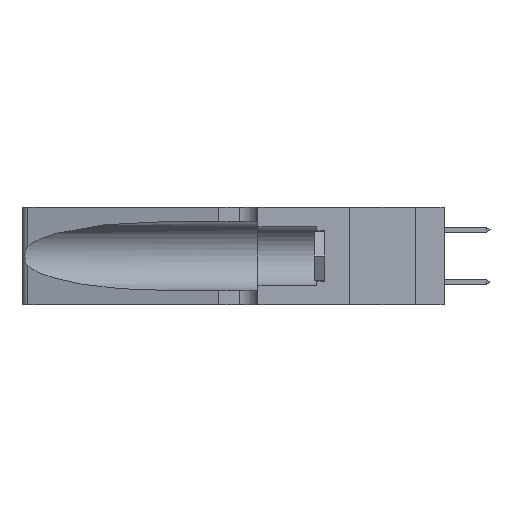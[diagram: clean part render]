
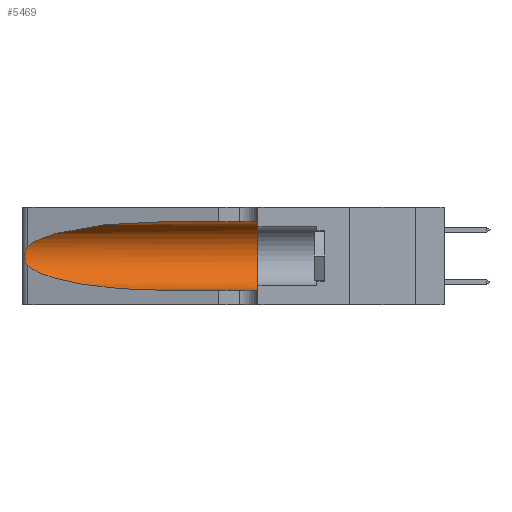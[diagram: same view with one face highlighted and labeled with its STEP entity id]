
A CAD part, left-side view. The second image highlights one B-rep face of the part: STEP entity #5469.
In plain terms, the highlighted cylindrical face has radius 3.308 mm (diameter 6.617 mm), a partial arc.
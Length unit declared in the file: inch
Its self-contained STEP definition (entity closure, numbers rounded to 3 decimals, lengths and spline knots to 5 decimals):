
#1336 = CARTESIAN_POINT ( 'NONE',  ( 0.1305, 1.61858, 0.185 ) ) ;
#1369 = ORIENTED_EDGE ( 'NONE', *, *, #7518, .T. ) ;
#2101 = DIRECTION ( 'NONE',  ( 0., -1., 0. ) ) ;
#2348 = EDGE_CURVE ( 'NONE', #13740, #12938, #23797, .T. ) ;
#2750 = CARTESIAN_POINT ( 'NONE',  ( 0.26018, 1.23835, 0.19895 ) ) ;
#2920 = CARTESIAN_POINT ( 'NONE',  ( 0.26017, 1.23833, 0.17102 ) ) ;
#3438 = CARTESIAN_POINT ( 'NONE',  ( 0.25487, 1.22718, 0.14631 ) ) ;
#4568 = EDGE_LOOP ( 'NONE', ( #7108, #1369, #13093, #8150, #4932, #17417 ) ) ;
#4824 = CARTESIAN_POINT ( 'NONE',  ( 0.25789, 1.23486, 0.15765 ) ) ;
#4932 = ORIENTED_EDGE ( 'NONE', *, *, #16822, .F. ) ;
#5037 = CARTESIAN_POINT ( 'NONE',  ( 0.25487, 1.22718, 0.22369 ) ) ;
#5038 = CARTESIAN_POINT ( 'NONE',  ( 0.1305, 0.72297, 0.05475 ) ) ;
#5103 = FACE_OUTER_BOUND ( 'NONE', #4568, .T. ) ;
#5469 = ADVANCED_FACE ( 'NONE', ( #5103 ), #8925, .F. ) ;
#5635 = DIRECTION ( 'NONE',  ( 0., -1., 0. ) ) ;
#6084 = VERTEX_POINT ( 'NONE', #10677 ) ;
#6521 = CARTESIAN_POINT ( 'NONE',  ( 0.25555, 1.22993, 0.14849 ) ) ;
#6771 = CARTESIAN_POINT ( 'NONE',  ( 0.25555, 1.22994, 0.2215 ) ) ;
#6838 = CARTESIAN_POINT ( 'NONE',  ( 0.1305, 0.35, 0.185 ) ) ;
#7108 = ORIENTED_EDGE ( 'NONE', *, *, #14461, .T. ) ;
#7281 = CARTESIAN_POINT ( 'NONE',  ( 0.25487, 1.22718, 0.22369 ) ) ;
#7518 = EDGE_CURVE ( 'NONE', #20914, #13740, #15071, .T. ) ;
#8150 = ORIENTED_EDGE ( 'NONE', *, *, #19286, .T. ) ;
#8511 = CARTESIAN_POINT ( 'NONE',  ( 0.18966, 0.96281, 0.31525 ) ) ;
#8925 = CYLINDRICAL_SURFACE ( 'NONE', #18607, 0.13025 ) ;
#10263 = CARTESIAN_POINT ( 'NONE',  ( 0.25487, 1.22718, 0.14631 ) ) ;
#10335 = AXIS2_PLACEMENT_3D ( 'NONE', #6838, #19932, #12716 ) ;
#10415 = CARTESIAN_POINT ( 'NONE',  ( 0.25854, 1.2359, 0.20912 ) ) ;
#10574 = CARTESIAN_POINT ( 'NONE',  ( 0.25639, 1.23184, 0.21858 ) ) ;
#10677 = CARTESIAN_POINT ( 'NONE',  ( 0.1305, 0.35, 0.05475 ) ) ;
#10706 = DIRECTION ( 'NONE',  ( 0., 0., -1. ) ) ;
#12007 = VERTEX_POINT ( 'NONE', #15693 ) ;
#12307 = CARTESIAN_POINT ( 'NONE',  ( 0.26075, 1.23896, 0.19203 ) ) ;
#12484 = CARTESIAN_POINT ( 'NONE',  ( 0.26075, 1.23896, 0.178 ) ) ;
#12716 = DIRECTION ( 'NONE',  ( 0., 0., 1. ) ) ;
#12938 = VERTEX_POINT ( 'NONE', #5038 ) ;
#13093 = ORIENTED_EDGE ( 'NONE', *, *, #2348, .T. ) ;
#13740 = VERTEX_POINT ( 'NONE', #3438 ) ;
#13821 = CIRCLE ( 'NONE', #10335, 0.13025 ) ;
#14421 = CARTESIAN_POINT ( 'NONE',  ( 0.18966, 0.96281, 0.05475 ) ) ;
#14461 = EDGE_CURVE ( 'NONE', #12007, #20914, #16277, .T. ) ;
#14545 = VECTOR ( 'NONE', #5635, 39.37008 ) ;
#15071 = B_SPLINE_CURVE_WITH_KNOTS ( 'NONE', 3,
 ( #21579, #6771, #10574, #23719, #10415, #2750, #12307, #12484, #2920, #23475, #4824, #23640, #6521, #10263 ),
 .UNSPECIFIED., .F., .F.,
 ( 4, 2, 2, 2, 2, 2, 4 ),
 ( 0., 0.00027, 0.00053, 0.00107, 0.0016, 0.00187, 0.00214 ),
 .UNSPECIFIED. ) ;
#15334 = VERTEX_POINT ( 'NONE', #21741 ) ;
#15693 = CARTESIAN_POINT ( 'NONE',  ( 0.1305, 0.72297, 0.31525 ) ) ;
#16277 =( BOUNDED_CURVE ( )  B_SPLINE_CURVE ( 3, ( #19763, #8511, #23928, #5037 ),
 .UNSPECIFIED., .F., .T. ) 
 B_SPLINE_CURVE_WITH_KNOTS ( ( 4, 4 ),
 ( 1.5708, 2.84003 ),
 .UNSPECIFIED. ) 
 CURVE ( )  GEOMETRIC_REPRESENTATION_ITEM ( )  RATIONAL_B_SPLINE_CURVE ( ( 1., 0.87, 0.87, 1. ) ) 
 REPRESENTATION_ITEM ( '' )  );
#16314 = CARTESIAN_POINT ( 'NONE',  ( 0.1305, 0.72297, 0.05475 ) ) ;
#16399 = VECTOR ( 'NONE', #2101, 39.37008 ) ;
#16822 = EDGE_CURVE ( 'NONE', #15334, #6084, #13821, .T. ) ;
#17417 = ORIENTED_EDGE ( 'NONE', *, *, #20610, .F. ) ;
#18607 = AXIS2_PLACEMENT_3D ( 'NONE', #1336, #20318, #10706 ) ;
#19286 = EDGE_CURVE ( 'NONE', #12938, #6084, #21358, .T. ) ;
#19531 = LINE ( 'NONE', #20537, #14545 ) ;
#19763 = CARTESIAN_POINT ( 'NONE',  ( 0.1305, 0.72297, 0.31525 ) ) ;
#19908 = CARTESIAN_POINT ( 'NONE',  ( 0.2373, 1.15595, 0.08982 ) ) ;
#19932 = DIRECTION ( 'NONE',  ( 0., 1., 0. ) ) ;
#20318 = DIRECTION ( 'NONE',  ( 0., -1., 0. ) ) ;
#20537 = CARTESIAN_POINT ( 'NONE',  ( 0.1305, 1.61858, 0.31525 ) ) ;
#20610 = EDGE_CURVE ( 'NONE', #12007, #15334, #19531, .T. ) ;
#20748 = CARTESIAN_POINT ( 'NONE',  ( 0.1305, 1.61858, 0.05475 ) ) ;
#20914 = VERTEX_POINT ( 'NONE', #7281 ) ;
#21358 = LINE ( 'NONE', #20748, #16399 ) ;
#21579 = CARTESIAN_POINT ( 'NONE',  ( 0.25487, 1.22718, 0.22369 ) ) ;
#21625 = CARTESIAN_POINT ( 'NONE',  ( 0.25487, 1.22718, 0.14631 ) ) ;
#21741 = CARTESIAN_POINT ( 'NONE',  ( 0.1305, 0.35, 0.31525 ) ) ;
#23475 = CARTESIAN_POINT ( 'NONE',  ( 0.25856, 1.23593, 0.16098 ) ) ;
#23640 = CARTESIAN_POINT ( 'NONE',  ( 0.25639, 1.23186, 0.15144 ) ) ;
#23719 = CARTESIAN_POINT ( 'NONE',  ( 0.25787, 1.23484, 0.2124 ) ) ;
#23797 =( BOUNDED_CURVE ( )  B_SPLINE_CURVE ( 3, ( #21625, #19908, #14421, #16314 ),
 .UNSPECIFIED., .F., .F. ) 
 B_SPLINE_CURVE_WITH_KNOTS ( ( 4, 4 ),
 ( 3.44316, 4.71239 ),
 .UNSPECIFIED. ) 
 CURVE ( )  GEOMETRIC_REPRESENTATION_ITEM ( )  RATIONAL_B_SPLINE_CURVE ( ( 1., 0.87, 0.87, 1. ) ) 
 REPRESENTATION_ITEM ( '' )  );
#23928 = CARTESIAN_POINT ( 'NONE',  ( 0.2373, 1.15595, 0.28018 ) ) ;
